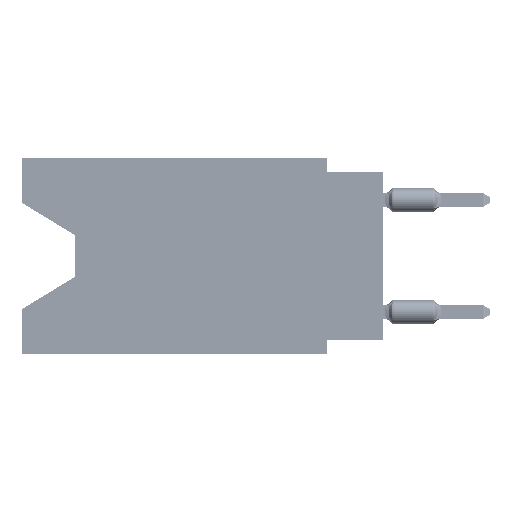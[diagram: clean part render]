
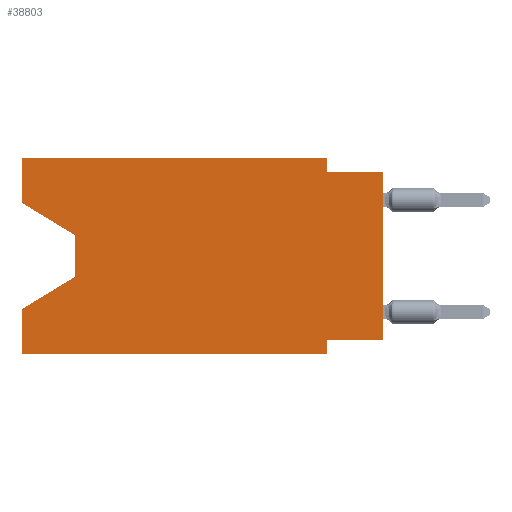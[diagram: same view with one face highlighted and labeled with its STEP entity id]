
A CAD part, left-side view. The second image highlights one B-rep face of the part: STEP entity #38803.
In plain terms, the highlighted planar face has unit normal (-1, 0, 0).
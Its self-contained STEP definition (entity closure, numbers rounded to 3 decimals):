
#355 = ORIENTED_EDGE ( 'NONE', *, *, #29703, .T. ) ;
#453 = ORIENTED_EDGE ( 'NONE', *, *, #4005, .F. ) ;
#772 = VECTOR ( 'NONE', #58371, 1000. ) ;
#1468 = CARTESIAN_POINT ( 'NONE',  ( 0., 16.383, 0. ) ) ;
#2726 = FACE_OUTER_BOUND ( 'NONE', #12988, .T. ) ;
#3180 = CARTESIAN_POINT ( 'NONE',  ( 0., 16.383, -2.038 ) ) ;
#3932 = CARTESIAN_POINT ( 'NONE',  ( 0., 2.54, 0. ) ) ;
#4005 = EDGE_CURVE ( 'NONE', #68838, #28706, #16409, .T. ) ;
#4639 = CARTESIAN_POINT ( 'NONE',  ( 0., 2.54, -8.89 ) ) ;
#5053 = EDGE_CURVE ( 'NONE', #36518, #23289, #21287, .T. ) ;
#6294 = LINE ( 'NONE', #81674, #39720 ) ;
#7510 = EDGE_CURVE ( 'NONE', #84453, #20563, #26494, .T. ) ;
#7729 = CARTESIAN_POINT ( 'NONE',  ( 0., 16.383, 0. ) ) ;
#8110 = VECTOR ( 'NONE', #65577, 1000. ) ;
#10081 = CARTESIAN_POINT ( 'NONE',  ( 0., 16.383, 0. ) ) ;
#10100 = LINE ( 'NONE', #45478, #81892 ) ;
#12091 = ORIENTED_EDGE ( 'NONE', *, *, #56465, .F. ) ;
#12338 = ORIENTED_EDGE ( 'NONE', *, *, #45715, .T. ) ;
#12988 = EDGE_LOOP ( 'NONE', ( #355, #26889, #80261, #45994, #74337, #12091, #86562, #12338, #453, #13656, #50753, #34141 ) ) ;
#13656 = ORIENTED_EDGE ( 'NONE', *, *, #54651, .F. ) ;
#14492 = CARTESIAN_POINT ( 'NONE',  ( 0., 13.97, -3.505 ) ) ;
#15345 = VERTEX_POINT ( 'NONE', #26636 ) ;
#16409 = LINE ( 'NONE', #17754, #8110 ) ;
#17209 = CARTESIAN_POINT ( 'NONE',  ( 0., 16.383, -2.038 ) ) ;
#17754 = CARTESIAN_POINT ( 'NONE',  ( 0., 0., -0.635 ) ) ;
#19778 = CARTESIAN_POINT ( 'NONE',  ( 0., 2.54, -8.255 ) ) ;
#20563 = VERTEX_POINT ( 'NONE', #7729 ) ;
#21287 = LINE ( 'NONE', #70892, #52256 ) ;
#23289 = VERTEX_POINT ( 'NONE', #50703 ) ;
#26023 = EDGE_CURVE ( 'NONE', #23289, #15345, #67080, .T. ) ;
#26494 = LINE ( 'NONE', #45824, #83181 ) ;
#26598 = LINE ( 'NONE', #90431, #86425 ) ;
#26636 = CARTESIAN_POINT ( 'NONE',  ( 0., 16.383, -6.852 ) ) ;
#26889 = ORIENTED_EDGE ( 'NONE', *, *, #5053, .T. ) ;
#28706 = VERTEX_POINT ( 'NONE', #69358 ) ;
#29703 = EDGE_CURVE ( 'NONE', #84453, #36518, #80142, .T. ) ;
#33200 = VERTEX_POINT ( 'NONE', #4639 ) ;
#33397 = DIRECTION ( 'NONE',  ( 0., 0., 1. ) ) ;
#34141 = ORIENTED_EDGE ( 'NONE', *, *, #7510, .F. ) ;
#36518 = VERTEX_POINT ( 'NONE', #14492 ) ;
#36523 = VERTEX_POINT ( 'NONE', #76984 ) ;
#36855 = LINE ( 'NONE', #73116, #58757 ) ;
#37012 = EDGE_CURVE ( 'NONE', #20563, #64811, #84654, .T. ) ;
#38123 = DIRECTION ( 'NONE',  ( 1., 0., 0. ) ) ;
#38803 = ADVANCED_FACE ( 'NONE', ( #2726 ), #78576, .F. ) ;
#39720 = VECTOR ( 'NONE', #48136, 1000. ) ;
#45242 = DIRECTION ( 'NONE',  ( 0., -0.855, -0.519 ) ) ;
#45415 = VERTEX_POINT ( 'NONE', #61189 ) ;
#45478 = CARTESIAN_POINT ( 'NONE',  ( 0., 0., -8.255 ) ) ;
#45586 = VECTOR ( 'NONE', #90630, 1000. ) ;
#45715 = EDGE_CURVE ( 'NONE', #36523, #28706, #59274, .T. ) ;
#45824 = CARTESIAN_POINT ( 'NONE',  ( 0., 16.383, 0. ) ) ;
#45994 = ORIENTED_EDGE ( 'NONE', *, *, #57992, .F. ) ;
#48136 = DIRECTION ( 'NONE',  ( 0., -1., 0. ) ) ;
#50703 = CARTESIAN_POINT ( 'NONE',  ( 0., 13.97, -5.385 ) ) ;
#50753 = ORIENTED_EDGE ( 'NONE', *, *, #37012, .F. ) ;
#52256 = VECTOR ( 'NONE', #76879, 1000. ) ;
#52370 = CARTESIAN_POINT ( 'NONE',  ( 0., 0., 0. ) ) ;
#52374 = DIRECTION ( 'NONE',  ( 0., 1., 0. ) ) ;
#53744 = EDGE_CURVE ( 'NONE', #36523, #65147, #10100, .T. ) ;
#54651 = EDGE_CURVE ( 'NONE', #64811, #68838, #26598, .T. ) ;
#56465 = EDGE_CURVE ( 'NONE', #65147, #33200, #36855, .T. ) ;
#57992 = EDGE_CURVE ( 'NONE', #45415, #15345, #78223, .T. ) ;
#58237 = VECTOR ( 'NONE', #45242, 1000. ) ;
#58371 = DIRECTION ( 'NONE',  ( 0., 0.855, -0.519 ) ) ;
#58757 = VECTOR ( 'NONE', #58885, 1000. ) ;
#58885 = DIRECTION ( 'NONE',  ( 0., 0., -1. ) ) ;
#59260 = DIRECTION ( 'NONE',  ( 0., 0., -1. ) ) ;
#59274 = LINE ( 'NONE', #52370, #80204 ) ;
#61189 = CARTESIAN_POINT ( 'NONE',  ( 0., 16.383, -8.89 ) ) ;
#62635 = DIRECTION ( 'NONE',  ( 0., 0., 1. ) ) ;
#62911 = DIRECTION ( 'NONE',  ( 0., 0., -1. ) ) ;
#64811 = VERTEX_POINT ( 'NONE', #3932 ) ;
#65147 = VERTEX_POINT ( 'NONE', #19778 ) ;
#65278 = CARTESIAN_POINT ( 'NONE',  ( 0., 13.97, -5.385 ) ) ;
#65577 = DIRECTION ( 'NONE',  ( 0., -1., 0. ) ) ;
#67080 = LINE ( 'NONE', #65278, #772 ) ;
#68838 = VERTEX_POINT ( 'NONE', #90049 ) ;
#69358 = CARTESIAN_POINT ( 'NONE',  ( 0., 0., -0.635 ) ) ;
#70495 = VECTOR ( 'NONE', #62635, 1000. ) ;
#70892 = CARTESIAN_POINT ( 'NONE',  ( 0., 13.97, -3.505 ) ) ;
#73116 = CARTESIAN_POINT ( 'NONE',  ( 0., 2.54, -8.89 ) ) ;
#74337 = ORIENTED_EDGE ( 'NONE', *, *, #81234, .T. ) ;
#76879 = DIRECTION ( 'NONE',  ( 0., 0., -1. ) ) ;
#76984 = CARTESIAN_POINT ( 'NONE',  ( 0., 0., -8.255 ) ) ;
#78223 = LINE ( 'NONE', #1468, #70495 ) ;
#78576 = PLANE ( 'NONE',  #79426 ) ;
#79426 = AXIS2_PLACEMENT_3D ( 'NONE', #10081, #38123, #59260 ) ;
#80142 = LINE ( 'NONE', #17209, #58237 ) ;
#80204 = VECTOR ( 'NONE', #80381, 1000. ) ;
#80261 = ORIENTED_EDGE ( 'NONE', *, *, #26023, .T. ) ;
#80381 = DIRECTION ( 'NONE',  ( 0., 0., 1. ) ) ;
#81234 = EDGE_CURVE ( 'NONE', #45415, #33200, #6294, .T. ) ;
#81674 = CARTESIAN_POINT ( 'NONE',  ( 0., 16.383, -8.89 ) ) ;
#81892 = VECTOR ( 'NONE', #52374, 1000. ) ;
#83181 = VECTOR ( 'NONE', #33397, 1000. ) ;
#84453 = VERTEX_POINT ( 'NONE', #3180 ) ;
#84654 = LINE ( 'NONE', #90170, #45586 ) ;
#86425 = VECTOR ( 'NONE', #62911, 1000. ) ;
#86562 = ORIENTED_EDGE ( 'NONE', *, *, #53744, .F. ) ;
#90049 = CARTESIAN_POINT ( 'NONE',  ( 0., 2.54, -0.635 ) ) ;
#90170 = CARTESIAN_POINT ( 'NONE',  ( 0., 16.383, 0. ) ) ;
#90431 = CARTESIAN_POINT ( 'NONE',  ( 0., 2.54, 0. ) ) ;
#90630 = DIRECTION ( 'NONE',  ( 0., -1., 0. ) ) ;
